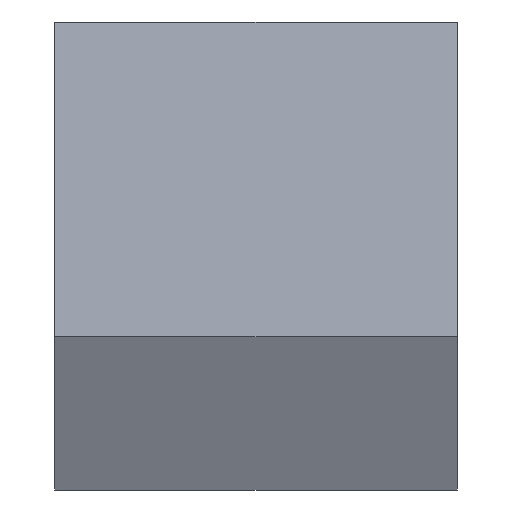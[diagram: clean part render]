
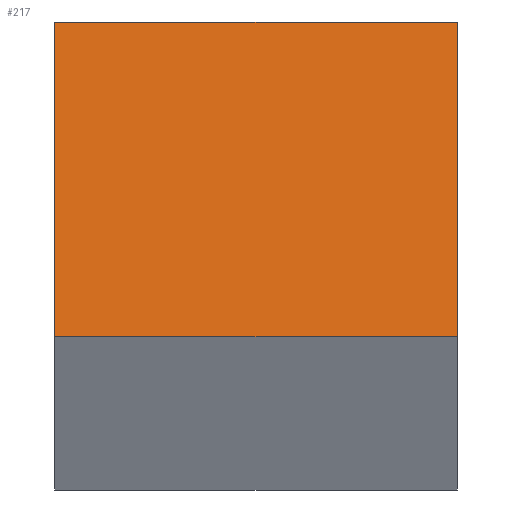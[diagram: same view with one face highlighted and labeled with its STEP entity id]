
A CAD part, top view. The second image highlights one B-rep face of the part: STEP entity #217.
In plain terms, the highlighted planar face has unit normal (0, 0.899, 0.438).
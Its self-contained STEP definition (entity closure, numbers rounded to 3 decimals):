
#83=CARTESIAN_POINT('',(9.5,-127.331,-213.417));
#84=VERTEX_POINT('',#83);
#91=CARTESIAN_POINT('',(-9.5,-127.331,-213.417));
#92=VERTEX_POINT('',#91);
#93=CARTESIAN_POINT('',(-9.5,-127.331,-213.417));
#94=DIRECTION('',(1.0,0.0,0.0));
#95=VECTOR('',#94,19.0);
#96=LINE('',#93,#95);
#97=EDGE_CURVE('',#92,#84,#96,.T.);
#139=CARTESIAN_POINT('',(9.5,-112.426,-243.976));
#140=VERTEX_POINT('',#139);
#147=CARTESIAN_POINT('',(9.5,-127.331,-213.417));
#148=DIRECTION('',(0.0,0.438,-0.899));
#149=VECTOR('',#148,34.);
#150=LINE('',#147,#149);
#151=EDGE_CURVE('',#84,#140,#150,.T.);
#171=CARTESIAN_POINT('',(-9.5,-112.426,-243.976));
#172=VERTEX_POINT('',#171);
#173=CARTESIAN_POINT('',(-9.5,-112.426,-243.976));
#174=DIRECTION('',(0.0,-0.438,0.899));
#175=VECTOR('',#174,34.);
#176=LINE('',#173,#175);
#177=EDGE_CURVE('',#172,#92,#176,.T.);
#201=CARTESIAN_POINT('',(0.0,-127.331,-213.417));
#202=DIRECTION('',(0.0,0.899,0.438));
#203=DIRECTION('',(0.0,-0.438,0.899));
#204=AXIS2_PLACEMENT_3D('',#201,#202,#203);
#205=PLANE('',#204);
#206=ORIENTED_EDGE('',*,*,#151,.T.);
#207=CARTESIAN_POINT('',(-9.5,-112.426,-243.976));
#208=DIRECTION('',(1.0,0.0,0.0));
#209=VECTOR('',#208,19.0);
#210=LINE('',#207,#209);
#211=EDGE_CURVE('',#172,#140,#210,.T.);
#212=ORIENTED_EDGE('',*,*,#211,.F.);
#213=ORIENTED_EDGE('',*,*,#177,.T.);
#214=ORIENTED_EDGE('',*,*,#97,.T.);
#215=EDGE_LOOP('',(#206,#212,#213,#214));
#216=FACE_OUTER_BOUND('',#215,.T.);
#217=ADVANCED_FACE('',(#216),#205,.T.);
